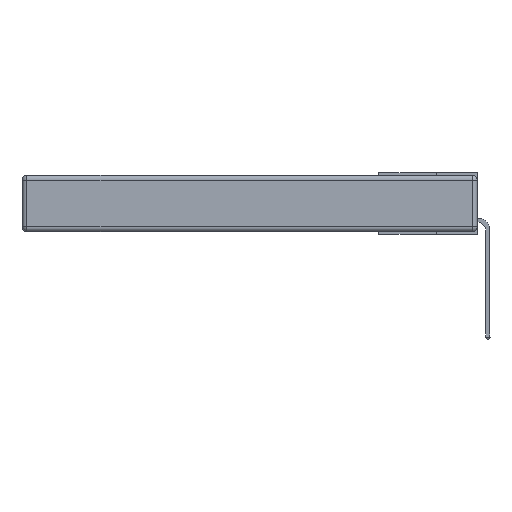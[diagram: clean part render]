
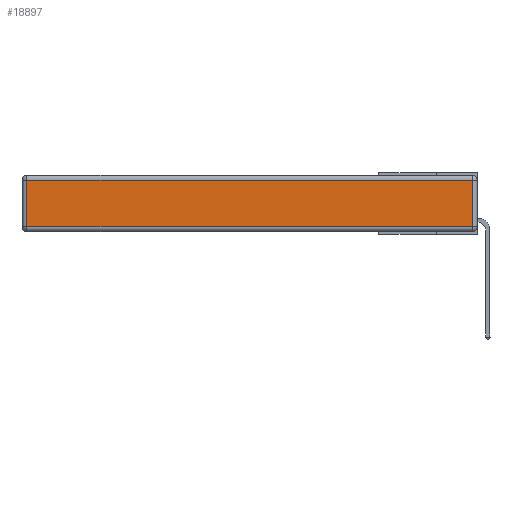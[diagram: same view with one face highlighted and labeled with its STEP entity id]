
A CAD part, left-side view. The second image highlights one B-rep face of the part: STEP entity #18897.
In plain terms, the highlighted planar face has unit normal (-1, 0, 0).
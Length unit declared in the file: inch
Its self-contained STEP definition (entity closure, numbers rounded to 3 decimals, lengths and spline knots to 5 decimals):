
#1401 = VECTOR ( 'NONE', #28548, 39.37008 ) ;
#3093 = CARTESIAN_POINT ( 'NONE',  ( 0., 0.03, -0.343 ) ) ;
#3348 = CARTESIAN_POINT ( 'NONE',  ( 0., 0., -0.343 ) ) ;
#4203 = CARTESIAN_POINT ( 'NONE',  ( 0., 2.72, -0.03 ) ) ;
#5611 = ORIENTED_EDGE ( 'NONE', *, *, #21294, .T. ) ;
#6224 = VECTOR ( 'NONE', #11366, 39.37008 ) ;
#6565 = LINE ( 'NONE', #21157, #1401 ) ;
#7051 = CARTESIAN_POINT ( 'NONE',  ( 0., 0.03, -0.313 ) ) ;
#11079 = VERTEX_POINT ( 'NONE', #15647 ) ;
#11269 = CARTESIAN_POINT ( 'NONE',  ( 0., 0., -0.313 ) ) ;
#11366 = DIRECTION ( 'NONE',  ( 0., -1., 0. ) ) ;
#11540 = EDGE_CURVE ( 'NONE', #17697, #19044, #22891, .T. ) ;
#12127 = LINE ( 'NONE', #11269, #6224 ) ;
#12453 = ORIENTED_EDGE ( 'NONE', *, *, #17311, .T. ) ;
#14149 = EDGE_LOOP ( 'NONE', ( #5611, #24789, #30048, #12453 ) ) ;
#14153 = CARTESIAN_POINT ( 'NONE',  ( 0., 2.75, -0.03 ) ) ;
#15647 = CARTESIAN_POINT ( 'NONE',  ( 0., 2.72, -0.313 ) ) ;
#17311 = EDGE_CURVE ( 'NONE', #29837, #11079, #6565, .T. ) ;
#17430 = VECTOR ( 'NONE', #20762, 39.37008 ) ;
#17697 = VERTEX_POINT ( 'NONE', #7051 ) ;
#18897 = ADVANCED_FACE ( 'NONE', ( #25541 ), #19322, .T. ) ;
#19044 = VERTEX_POINT ( 'NONE', #27181 ) ;
#19322 = PLANE ( 'NONE',  #19375 ) ;
#19375 = AXIS2_PLACEMENT_3D ( 'NONE', #3348, #21567, #21674 ) ;
#19696 = EDGE_CURVE ( 'NONE', #19044, #29837, #21447, .T. ) ;
#20762 = DIRECTION ( 'NONE',  ( 0., 1., 0. ) ) ;
#21157 = CARTESIAN_POINT ( 'NONE',  ( 0., 2.72, -0.343 ) ) ;
#21294 = EDGE_CURVE ( 'NONE', #11079, #17697, #12127, .T. ) ;
#21447 = LINE ( 'NONE', #14153, #17430 ) ;
#21567 = DIRECTION ( 'NONE',  ( -1., 0., 0. ) ) ;
#21674 = DIRECTION ( 'NONE',  ( 0., 0., 1. ) ) ;
#22891 = LINE ( 'NONE', #3093, #23620 ) ;
#23093 = DIRECTION ( 'NONE',  ( 0., 0., 1. ) ) ;
#23620 = VECTOR ( 'NONE', #23093, 39.37008 ) ;
#24789 = ORIENTED_EDGE ( 'NONE', *, *, #11540, .T. ) ;
#25541 = FACE_OUTER_BOUND ( 'NONE', #14149, .T. ) ;
#27181 = CARTESIAN_POINT ( 'NONE',  ( 0., 0.03, -0.03 ) ) ;
#28548 = DIRECTION ( 'NONE',  ( 0., 0., -1. ) ) ;
#29837 = VERTEX_POINT ( 'NONE', #4203 ) ;
#30048 = ORIENTED_EDGE ( 'NONE', *, *, #19696, .T. ) ;
